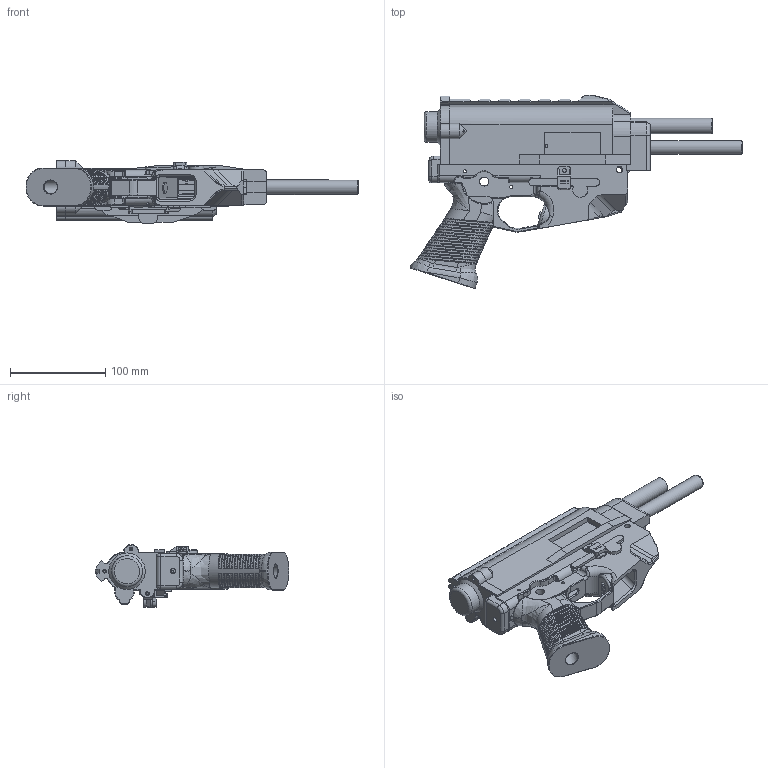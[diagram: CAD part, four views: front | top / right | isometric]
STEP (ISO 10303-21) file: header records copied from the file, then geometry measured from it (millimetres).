
FILE_DESCRIPTION(/* description */ ('','CAx-IF Rec.Pracs.---Representation and Presentation of Product Manufacturing Information (PMI)---3.8---2014-02-18'),/* implementation_level */ '2;1');
FILE_NAME(/* name */ 'WTF-9H full assembly v1.2.stp',/* time_stamp */ '2020-05-13T19:38:40-07:00',/* author */ ('Uber Lobster'),/* organization */ (''),/* preprocessor_version */ 'ST-DEVELOPER v16.13',/* originating_system */ 'Autodesk Inventor 2018',/* authorisation */ '');
FILE_SCHEMA (('AP242_MANAGED_MODEL_BASED_3D_ENGINEERING_MIM_LF { 1 0 10303 442 1 1 4 }'));
Products named in the file (22): WTF-9H full ass; WTF-9H_barrel_retainer; WTF HILLBILLY FINAL_9; WTF-9H_bolt_housing; WTF HILLBILLY FINAL_13; WTF-9H_ejector; WTF HILLBILLY FINAL_3; WTF-9H_ejector_mount; WTF HILLBILLY FINAL_11; WTF-9H_upper_receiver; Lower Bolt; WTF-9H_endcap; WTF HILLBILLY FINAL_5; WTF-9H_lower_receiver; WTF-9H_mag_catch; WTF-9H_mag_release_pivot_pin; WTF-9H_pistol_grip; WTF-9MV_mag_catch_mount; WTF9 V1 FINAL_7; Mag Button; Glock 9mm long barrel; Upper bolt
Assembly tree (21 placements, depth 3):
  WTF-9H full ass
    WTF-9H_barrel_retainer
      WTF HILLBILLY FINAL_9
    WTF-9H_bolt_housing
      WTF HILLBILLY FINAL_13
    WTF-9H_ejector
      WTF HILLBILLY FINAL_3
    WTF-9H_ejector_mount
      WTF HILLBILLY FINAL_11
    WTF-9H_upper_receiver
    Lower Bolt
    WTF-9H_endcap
      WTF HILLBILLY FINAL_5
    WTF-9H_lower_receiver
    WTF-9H_mag_catch
    WTF-9H_mag_release_pivot_pin
    WTF-9H_pistol_grip
    WTF-9MV_mag_catch_mount
      WTF9 V1 FINAL_7
    Mag Button
    Glock 9mm long barrel
    Upper bolt
Bounding box: 349.07 x 203.42 x 66.2 mm (x, y, z)
Volume: 772495 mm3; surface area: 247747.4 mm2
Topology: 16 solids, 21 shells, 2029 faces, 5516 edges, 3531 vertices
Faces by surface type: plane 1110, bspline 420, cylinder 392, torus 71, cone 32, sphere 4
Full cylindrical faces by diameter (mm): 2 x1, 2.2 x1, 2.4 x5, 2.5 x3, 2.6 x2, 2.968 x2, 3 x2, 3.175 x4, 3.469 x4, 3.5 x5, 3.566 x1, 3.7 x3, 3.962 x1, 4 x3, 5.105 x1, 5.5 x1, 5.8 x1, 5.9 x1, 6 x2, 6.2 x1, 6.34 x1, 6.375 x2, 6.4 x2, 7.8 x1, 8 x2, 9.525 x2, 12 x1, 14 x1, 14.5 x1, 16.2 x1
Entity records: 91918 total; most frequent: CARTESIAN_POINT 41011, ORIENTED_EDGE 10738, DIRECTION 9459, EDGE_CURVE 5365, VERTEX_POINT 3497, LINE 3481, VECTOR 3481, AXIS2_PLACEMENT_3D 3049
